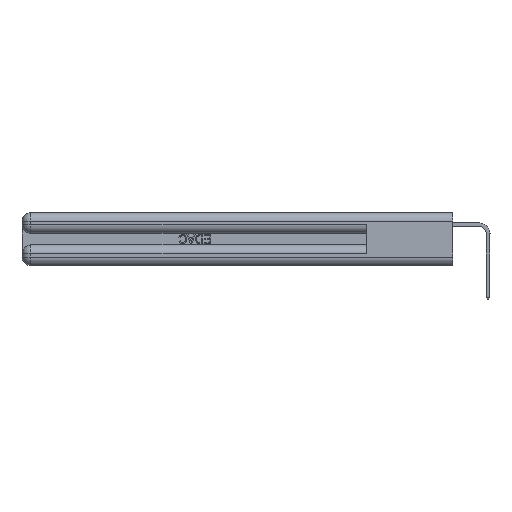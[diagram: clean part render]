
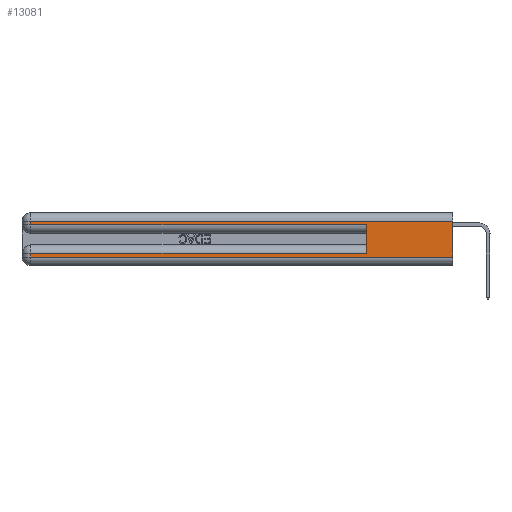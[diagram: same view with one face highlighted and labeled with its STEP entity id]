
A CAD part, left-side view. The second image highlights one B-rep face of the part: STEP entity #13081.
In plain terms, the highlighted planar face has unit normal (-1, 0, 0).
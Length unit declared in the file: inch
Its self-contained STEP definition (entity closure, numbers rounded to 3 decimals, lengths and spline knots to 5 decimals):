
#1465 = VERTEX_POINT ( 'NONE', #47770 ) ;
#1488 = VECTOR ( 'NONE', #41430, 39.37008 ) ;
#1608 = DIRECTION ( 'NONE',  ( 1., 0., 0. ) ) ;
#2136 = CARTESIAN_POINT ( 'NONE',  ( 0., 0., 0.285 ) ) ;
#2138 = LINE ( 'NONE', #47276, #21957 ) ;
#2954 = ORIENTED_EDGE ( 'NONE', *, *, #26567, .T. ) ;
#3518 = LINE ( 'NONE', #26358, #33133 ) ;
#5037 = VERTEX_POINT ( 'NONE', #18759 ) ;
#5671 = EDGE_CURVE ( 'NONE', #45435, #33183, #38076, .T. ) ;
#5712 = VECTOR ( 'NONE', #28741, 39.37008 ) ;
#5863 = DIRECTION ( 'NONE',  ( 0., -1., 0. ) ) ;
#7672 = ORIENTED_EDGE ( 'NONE', *, *, #5671, .T. ) ;
#8134 = AXIS2_PLACEMENT_3D ( 'NONE', #42299, #1608, #27623 ) ;
#10580 = DIRECTION ( 'NONE',  ( 0., 0., -1. ) ) ;
#10595 = CARTESIAN_POINT ( 'NONE',  ( 0., 2.94, 0.085 ) ) ;
#11586 = EDGE_CURVE ( 'NONE', #28901, #1465, #2138, .T. ) ;
#13081 = ADVANCED_FACE ( 'NONE', ( #16614 ), #38575, .F. ) ;
#15104 = CARTESIAN_POINT ( 'NONE',  ( 0., 0., 0.085 ) ) ;
#15246 = ORIENTED_EDGE ( 'NONE', *, *, #20663, .T. ) ;
#15546 = CARTESIAN_POINT ( 'NONE',  ( 0., 0., 0.06 ) ) ;
#16614 = FACE_OUTER_BOUND ( 'NONE', #17866, .T. ) ;
#16907 = ORIENTED_EDGE ( 'NONE', *, *, #11586, .T. ) ;
#17402 = CARTESIAN_POINT ( 'NONE',  ( 0., 2.94, 0.37 ) ) ;
#17682 = VECTOR ( 'NONE', #10580, 39.37008 ) ;
#17866 = EDGE_LOOP ( 'NONE', ( #34189, #16907, #46963, #2954, #22236, #7672, #21732, #15246 ) ) ;
#18160 = EDGE_CURVE ( 'NONE', #33183, #5037, #31265, .T. ) ;
#18759 = CARTESIAN_POINT ( 'NONE',  ( 0., 2.94, 0.06 ) ) ;
#19588 = VECTOR ( 'NONE', #40999, 39.37008 ) ;
#20238 = CARTESIAN_POINT ( 'NONE',  ( 0., 2.94, 0.285 ) ) ;
#20663 = EDGE_CURVE ( 'NONE', #5037, #28116, #40937, .T. ) ;
#21467 = DIRECTION ( 'NONE',  ( 0., 1., 0. ) ) ;
#21604 = EDGE_CURVE ( 'NONE', #1465, #36472, #47179, .T. ) ;
#21732 = ORIENTED_EDGE ( 'NONE', *, *, #18160, .T. ) ;
#21957 = VECTOR ( 'NONE', #21467, 39.37008 ) ;
#22236 = ORIENTED_EDGE ( 'NONE', *, *, #41392, .F. ) ;
#24367 = LINE ( 'NONE', #25037, #5712 ) ;
#25037 = CARTESIAN_POINT ( 'NONE',  ( 0., 0.6, 0.145 ) ) ;
#26358 = CARTESIAN_POINT ( 'NONE',  ( 0., 0., 0.37 ) ) ;
#26567 = EDGE_CURVE ( 'NONE', #36472, #27342, #47061, .T. ) ;
#27342 = VERTEX_POINT ( 'NONE', #46384 ) ;
#27623 = DIRECTION ( 'NONE',  ( 0., 0., -1. ) ) ;
#28116 = VERTEX_POINT ( 'NONE', #40062 ) ;
#28741 = DIRECTION ( 'NONE',  ( 0., 0., 1. ) ) ;
#28901 = VERTEX_POINT ( 'NONE', #37695 ) ;
#28970 = VECTOR ( 'NONE', #43275, 39.37008 ) ;
#30184 = DIRECTION ( 'NONE',  ( 0., 0., -1. ) ) ;
#31265 = LINE ( 'NONE', #17402, #28970 ) ;
#32800 = CARTESIAN_POINT ( 'NONE',  ( 0., 2.94, 0.37 ) ) ;
#33125 = CARTESIAN_POINT ( 'NONE',  ( 0., 0.6, 0.085 ) ) ;
#33133 = VECTOR ( 'NONE', #30184, 39.37008 ) ;
#33183 = VERTEX_POINT ( 'NONE', #10595 ) ;
#34189 = ORIENTED_EDGE ( 'NONE', *, *, #47258, .F. ) ;
#36472 = VERTEX_POINT ( 'NONE', #20238 ) ;
#37218 = VECTOR ( 'NONE', #5863, 39.37008 ) ;
#37695 = CARTESIAN_POINT ( 'NONE',  ( 0., 0., 0.31 ) ) ;
#38076 = LINE ( 'NONE', #15104, #19588 ) ;
#38575 = PLANE ( 'NONE',  #8134 ) ;
#40062 = CARTESIAN_POINT ( 'NONE',  ( 0., 0., 0.06 ) ) ;
#40937 = LINE ( 'NONE', #15546, #1488 ) ;
#40999 = DIRECTION ( 'NONE',  ( 0., 1., 0. ) ) ;
#41392 = EDGE_CURVE ( 'NONE', #45435, #27342, #24367, .T. ) ;
#41430 = DIRECTION ( 'NONE',  ( 0., -1., 0. ) ) ;
#42299 = CARTESIAN_POINT ( 'NONE',  ( 0., 0., 0.37 ) ) ;
#43275 = DIRECTION ( 'NONE',  ( 0., 0., -1. ) ) ;
#45435 = VERTEX_POINT ( 'NONE', #33125 ) ;
#46384 = CARTESIAN_POINT ( 'NONE',  ( 0., 0.6, 0.285 ) ) ;
#46963 = ORIENTED_EDGE ( 'NONE', *, *, #21604, .T. ) ;
#47061 = LINE ( 'NONE', #2136, #37218 ) ;
#47179 = LINE ( 'NONE', #32800, #17682 ) ;
#47258 = EDGE_CURVE ( 'NONE', #28901, #28116, #3518, .T. ) ;
#47276 = CARTESIAN_POINT ( 'NONE',  ( 0., 0., 0.31 ) ) ;
#47770 = CARTESIAN_POINT ( 'NONE',  ( 0., 2.94, 0.31 ) ) ;
